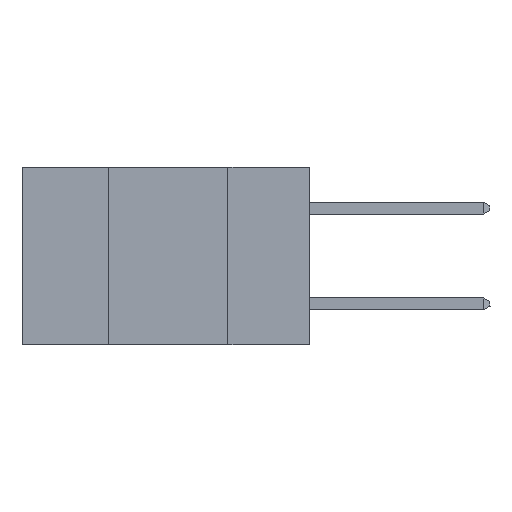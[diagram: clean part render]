
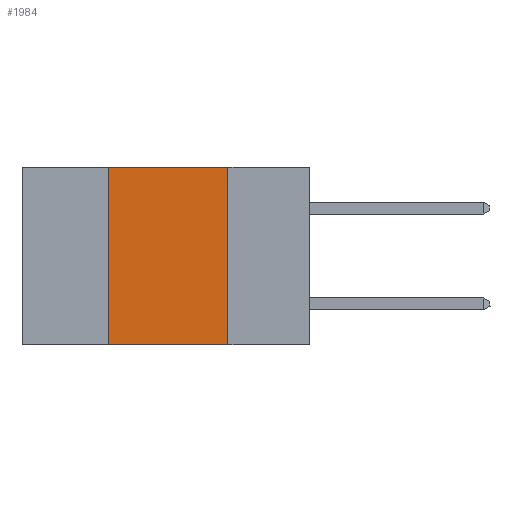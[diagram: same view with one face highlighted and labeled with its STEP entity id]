
A CAD part, left-side view. The second image highlights one B-rep face of the part: STEP entity #1984.
In plain terms, the highlighted planar face has unit normal (-1, 0, 0).
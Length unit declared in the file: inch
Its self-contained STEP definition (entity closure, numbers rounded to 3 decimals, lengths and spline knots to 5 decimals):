
#172 = DIRECTION ( 'NONE',  ( 0., 0., -1. ) ) ;
#321 = EDGE_LOOP ( 'NONE', ( #16051, #9071, #16560, #3661 ) ) ;
#969 = CARTESIAN_POINT ( 'NONE',  ( 0., 0.6, 0. ) ) ;
#994 = VERTEX_POINT ( 'NONE', #7701 ) ;
#1214 = LINE ( 'NONE', #8173, #14695 ) ;
#1235 = LINE ( 'NONE', #969, #3627 ) ;
#1625 = VERTEX_POINT ( 'NONE', #13705 ) ;
#1984 = ADVANCED_FACE ( 'NONE', ( #15959 ), #2945, .F. ) ;
#2032 = DIRECTION ( 'NONE',  ( 0., 0., -1. ) ) ;
#2174 = VECTOR ( 'NONE', #9365, 39.37008 ) ;
#2543 = EDGE_CURVE ( 'NONE', #10734, #15886, #9238, .T. ) ;
#2945 = PLANE ( 'NONE',  #15053 ) ;
#3627 = VECTOR ( 'NONE', #3812, 39.37008 ) ;
#3661 = ORIENTED_EDGE ( 'NONE', *, *, #10283, .T. ) ;
#3812 = DIRECTION ( 'NONE',  ( 0., -1., 0. ) ) ;
#4268 = DIRECTION ( 'NONE',  ( 0., -1., 0. ) ) ;
#5206 = CARTESIAN_POINT ( 'NONE',  ( 0., 0.6, 0. ) ) ;
#5740 = DIRECTION ( 'NONE',  ( 1., 0., 0. ) ) ;
#6062 = CARTESIAN_POINT ( 'NONE',  ( 0., 0.42, 0. ) ) ;
#7701 = CARTESIAN_POINT ( 'NONE',  ( 0., 0.17, 0. ) ) ;
#8144 = CARTESIAN_POINT ( 'NONE',  ( 0., 0.42, 0. ) ) ;
#8173 = CARTESIAN_POINT ( 'NONE',  ( 0., 0.6, -0.37 ) ) ;
#9071 = ORIENTED_EDGE ( 'NONE', *, *, #14999, .F. ) ;
#9238 = LINE ( 'NONE', #6062, #2174 ) ;
#9365 = DIRECTION ( 'NONE',  ( 0., 0., 1. ) ) ;
#10283 = EDGE_CURVE ( 'NONE', #10734, #1625, #1214, .T. ) ;
#10734 = VERTEX_POINT ( 'NONE', #15327 ) ;
#12813 = EDGE_CURVE ( 'NONE', #994, #1625, #16378, .T. ) ;
#13705 = CARTESIAN_POINT ( 'NONE',  ( 0., 0.17, -0.37 ) ) ;
#14695 = VECTOR ( 'NONE', #4268, 39.37008 ) ;
#14999 = EDGE_CURVE ( 'NONE', #15886, #994, #1235, .T. ) ;
#15053 = AXIS2_PLACEMENT_3D ( 'NONE', #5206, #5740, #2032 ) ;
#15327 = CARTESIAN_POINT ( 'NONE',  ( 0., 0.42, -0.37 ) ) ;
#15592 = VECTOR ( 'NONE', #172, 39.37008 ) ;
#15834 = CARTESIAN_POINT ( 'NONE',  ( 0., 0.17, 0. ) ) ;
#15886 = VERTEX_POINT ( 'NONE', #8144 ) ;
#15959 = FACE_OUTER_BOUND ( 'NONE', #321, .T. ) ;
#16051 = ORIENTED_EDGE ( 'NONE', *, *, #12813, .F. ) ;
#16378 = LINE ( 'NONE', #15834, #15592 ) ;
#16560 = ORIENTED_EDGE ( 'NONE', *, *, #2543, .F. ) ;
